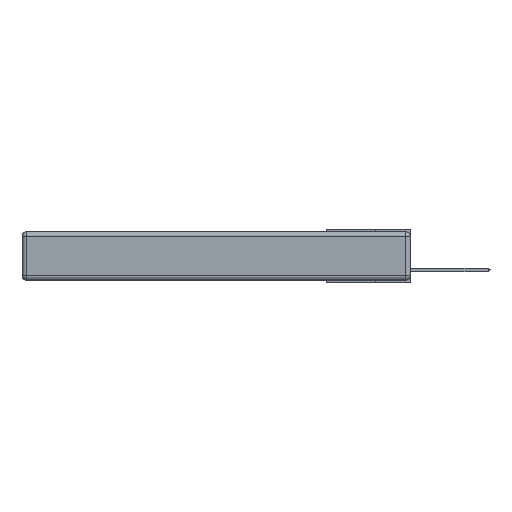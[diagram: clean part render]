
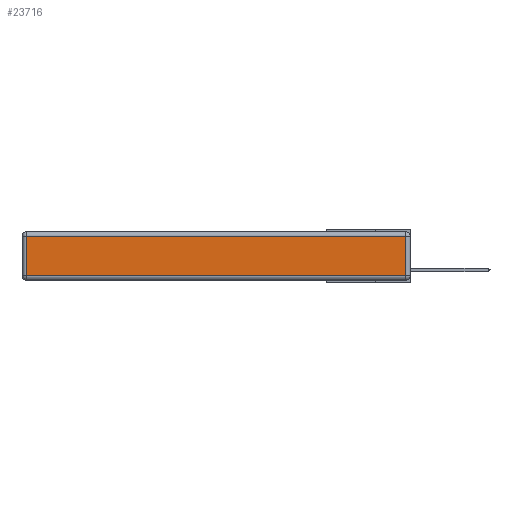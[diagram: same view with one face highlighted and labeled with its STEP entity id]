
A CAD part, left-side view. The second image highlights one B-rep face of the part: STEP entity #23716.
In plain terms, the highlighted planar face has unit normal (-1, 0, 0).
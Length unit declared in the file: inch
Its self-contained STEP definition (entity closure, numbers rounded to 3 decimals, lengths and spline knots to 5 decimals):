
#1336 = AXIS2_PLACEMENT_3D ( 'NONE', #25481, #16478, #20754 ) ;
#1804 = DIRECTION ( 'NONE',  ( 0., 0., -1. ) ) ;
#1861 = EDGE_CURVE ( 'NONE', #22038, #21200, #22234, .T. ) ;
#3426 = ORIENTED_EDGE ( 'NONE', *, *, #9702, .T. ) ;
#4212 = ORIENTED_EDGE ( 'NONE', *, *, #1861, .T. ) ;
#4237 = CARTESIAN_POINT ( 'NONE',  ( 0., 0.03, -0.03 ) ) ;
#4697 = PLANE ( 'NONE',  #1336 ) ;
#7820 = EDGE_CURVE ( 'NONE', #15011, #22038, #29338, .T. ) ;
#9702 = EDGE_CURVE ( 'NONE', #27398, #15011, #11736, .T. ) ;
#9824 = ORIENTED_EDGE ( 'NONE', *, *, #10526, .T. ) ;
#10526 = EDGE_CURVE ( 'NONE', #21200, #27398, #29201, .T. ) ;
#10574 = VECTOR ( 'NONE', #16983, 39.37008 ) ;
#10942 = CARTESIAN_POINT ( 'NONE',  ( 0., 2.72, -0.343 ) ) ;
#11736 = LINE ( 'NONE', #10942, #14974 ) ;
#12515 = CARTESIAN_POINT ( 'NONE',  ( 0., 0.03, -0.313 ) ) ;
#14974 = VECTOR ( 'NONE', #1804, 39.37008 ) ;
#15011 = VERTEX_POINT ( 'NONE', #16968 ) ;
#15093 = VECTOR ( 'NONE', #17656, 39.37008 ) ;
#16478 = DIRECTION ( 'NONE',  ( -1., 0., 0. ) ) ;
#16918 = DIRECTION ( 'NONE',  ( 0., 0., 1. ) ) ;
#16968 = CARTESIAN_POINT ( 'NONE',  ( 0., 2.72, -0.313 ) ) ;
#16983 = DIRECTION ( 'NONE',  ( 0., 1., 0. ) ) ;
#17217 = CARTESIAN_POINT ( 'NONE',  ( 0., 0.03, -0.343 ) ) ;
#17557 = CARTESIAN_POINT ( 'NONE',  ( 0., 0., -0.313 ) ) ;
#17656 = DIRECTION ( 'NONE',  ( 0., -1., 0. ) ) ;
#19129 = CARTESIAN_POINT ( 'NONE',  ( 0., 2.75, -0.03 ) ) ;
#20754 = DIRECTION ( 'NONE',  ( 0., 0., 1. ) ) ;
#20802 = VECTOR ( 'NONE', #16918, 39.37008 ) ;
#21030 = CARTESIAN_POINT ( 'NONE',  ( 0., 2.72, -0.03 ) ) ;
#21053 = FACE_OUTER_BOUND ( 'NONE', #25367, .T. ) ;
#21200 = VERTEX_POINT ( 'NONE', #4237 ) ;
#22038 = VERTEX_POINT ( 'NONE', #12515 ) ;
#22234 = LINE ( 'NONE', #17217, #20802 ) ;
#23716 = ADVANCED_FACE ( 'NONE', ( #21053 ), #4697, .T. ) ;
#24069 = ORIENTED_EDGE ( 'NONE', *, *, #7820, .T. ) ;
#25367 = EDGE_LOOP ( 'NONE', ( #24069, #4212, #9824, #3426 ) ) ;
#25481 = CARTESIAN_POINT ( 'NONE',  ( 0., 0., -0.343 ) ) ;
#27398 = VERTEX_POINT ( 'NONE', #21030 ) ;
#29201 = LINE ( 'NONE', #19129, #10574 ) ;
#29338 = LINE ( 'NONE', #17557, #15093 ) ;
